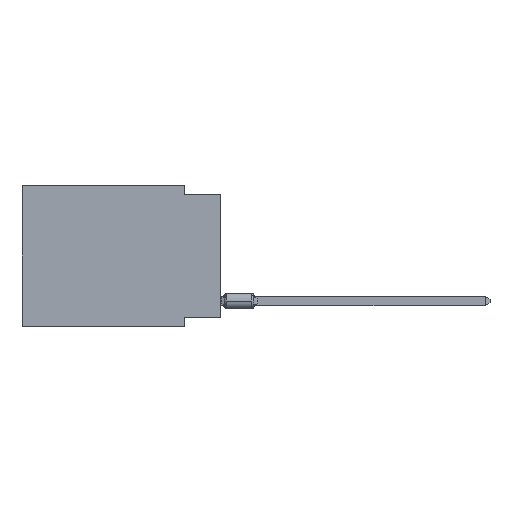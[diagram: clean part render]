
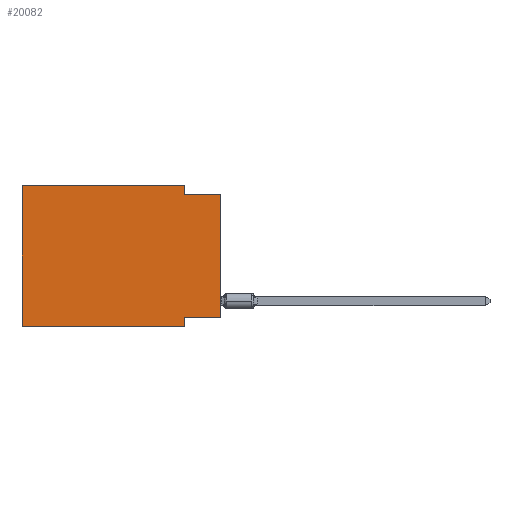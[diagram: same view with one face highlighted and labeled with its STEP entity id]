
A CAD part, left-side view. The second image highlights one B-rep face of the part: STEP entity #20082.
In plain terms, the highlighted planar face has unit normal (-1, 0, 0).
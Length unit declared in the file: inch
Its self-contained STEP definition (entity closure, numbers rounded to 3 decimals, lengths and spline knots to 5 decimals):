
#296 = VERTEX_POINT ( 'NONE', #24449 ) ;
#1430 = CARTESIAN_POINT ( 'NONE',  ( 0., 0.55, 0. ) ) ;
#1585 = ORIENTED_EDGE ( 'NONE', *, *, #33743, .F. ) ;
#2150 = CARTESIAN_POINT ( 'NONE',  ( 0., 0.1, -0.39 ) ) ;
#3085 = LINE ( 'NONE', #27768, #36129 ) ;
#3316 = ORIENTED_EDGE ( 'NONE', *, *, #31457, .F. ) ;
#4419 = CARTESIAN_POINT ( 'NONE',  ( 0., 0., -0.025 ) ) ;
#4659 = DIRECTION ( 'NONE',  ( 1., 0., 0. ) ) ;
#4661 = EDGE_CURVE ( 'NONE', #14690, #7170, #20690, .T. ) ;
#6066 = EDGE_CURVE ( 'NONE', #33749, #36734, #11482, .T. ) ;
#6223 = LINE ( 'NONE', #31396, #40293 ) ;
#7170 = VERTEX_POINT ( 'NONE', #2150 ) ;
#8730 = EDGE_LOOP ( 'NONE', ( #40315, #3316, #1585, #43874, #40571, #9997, #23531, #31334 ) ) ;
#8851 = DIRECTION ( 'NONE',  ( 0., 0., -1. ) ) ;
#9298 = LINE ( 'NONE', #12766, #36485 ) ;
#9997 = ORIENTED_EDGE ( 'NONE', *, *, #4661, .T. ) ;
#10073 = DIRECTION ( 'NONE',  ( 0., -1., 0. ) ) ;
#10293 = CARTESIAN_POINT ( 'NONE',  ( 0., 0.1, -0.365 ) ) ;
#11482 = LINE ( 'NONE', #38988, #27968 ) ;
#11809 = CARTESIAN_POINT ( 'NONE',  ( 0., 0., -0.365 ) ) ;
#12328 = VECTOR ( 'NONE', #10073, 39.37008 ) ;
#12766 = CARTESIAN_POINT ( 'NONE',  ( 0., 0.1, -0.39 ) ) ;
#13366 = CARTESIAN_POINT ( 'NONE',  ( 0., 0.1, 0. ) ) ;
#13675 = DIRECTION ( 'NONE',  ( 0., 0., -1. ) ) ;
#14138 = CARTESIAN_POINT ( 'NONE',  ( 0., 0.55, 0. ) ) ;
#14594 = FACE_OUTER_BOUND ( 'NONE', #8730, .T. ) ;
#14690 = VERTEX_POINT ( 'NONE', #22572 ) ;
#15009 = AXIS2_PLACEMENT_3D ( 'NONE', #1430, #4659, #25920 ) ;
#16118 = VERTEX_POINT ( 'NONE', #10293 ) ;
#18656 = LINE ( 'NONE', #36907, #40314 ) ;
#20082 = ADVANCED_FACE ( 'NONE', ( #14594 ), #32139, .F. ) ;
#20690 = LINE ( 'NONE', #31981, #36551 ) ;
#20991 = DIRECTION ( 'NONE',  ( 0., 0., 1. ) ) ;
#21405 = CARTESIAN_POINT ( 'NONE',  ( 0., 0., -0.025 ) ) ;
#22572 = CARTESIAN_POINT ( 'NONE',  ( 0., 0.55, -0.39 ) ) ;
#23531 = ORIENTED_EDGE ( 'NONE', *, *, #25325, .F. ) ;
#23603 = EDGE_CURVE ( 'NONE', #39385, #16118, #18656, .T. ) ;
#24449 = CARTESIAN_POINT ( 'NONE',  ( 0., 0.1, -0.025 ) ) ;
#25109 = LINE ( 'NONE', #21405, #12328 ) ;
#25325 = EDGE_CURVE ( 'NONE', #16118, #7170, #9298, .T. ) ;
#25920 = DIRECTION ( 'NONE',  ( 0., 0., -1. ) ) ;
#26837 = CARTESIAN_POINT ( 'NONE',  ( 0., 0.55, 0. ) ) ;
#27135 = VERTEX_POINT ( 'NONE', #4419 ) ;
#27327 = EDGE_CURVE ( 'NONE', #39385, #27135, #6223, .T. ) ;
#27741 = LINE ( 'NONE', #26837, #38940 ) ;
#27768 = CARTESIAN_POINT ( 'NONE',  ( 0., 0.1, 0. ) ) ;
#27968 = VECTOR ( 'NONE', #28587, 39.37008 ) ;
#28587 = DIRECTION ( 'NONE',  ( 0., -1., 0. ) ) ;
#30510 = EDGE_CURVE ( 'NONE', #14690, #33749, #27741, .T. ) ;
#31334 = ORIENTED_EDGE ( 'NONE', *, *, #23603, .F. ) ;
#31396 = CARTESIAN_POINT ( 'NONE',  ( 0., 0., 0. ) ) ;
#31457 = EDGE_CURVE ( 'NONE', #296, #27135, #25109, .T. ) ;
#31981 = CARTESIAN_POINT ( 'NONE',  ( 0., 0.55, -0.39 ) ) ;
#32139 = PLANE ( 'NONE',  #15009 ) ;
#33743 = EDGE_CURVE ( 'NONE', #36734, #296, #3085, .T. ) ;
#33749 = VERTEX_POINT ( 'NONE', #14138 ) ;
#36129 = VECTOR ( 'NONE', #13675, 39.37008 ) ;
#36485 = VECTOR ( 'NONE', #8851, 39.37008 ) ;
#36551 = VECTOR ( 'NONE', #41936, 39.37008 ) ;
#36734 = VERTEX_POINT ( 'NONE', #13366 ) ;
#36907 = CARTESIAN_POINT ( 'NONE',  ( 0., 0., -0.365 ) ) ;
#38940 = VECTOR ( 'NONE', #44849, 39.37008 ) ;
#38988 = CARTESIAN_POINT ( 'NONE',  ( 0., 0.55, 0. ) ) ;
#39385 = VERTEX_POINT ( 'NONE', #11809 ) ;
#40293 = VECTOR ( 'NONE', #20991, 39.37008 ) ;
#40314 = VECTOR ( 'NONE', #43140, 39.37008 ) ;
#40315 = ORIENTED_EDGE ( 'NONE', *, *, #27327, .T. ) ;
#40571 = ORIENTED_EDGE ( 'NONE', *, *, #30510, .F. ) ;
#41936 = DIRECTION ( 'NONE',  ( 0., -1., 0. ) ) ;
#43140 = DIRECTION ( 'NONE',  ( 0., 1., 0. ) ) ;
#43874 = ORIENTED_EDGE ( 'NONE', *, *, #6066, .F. ) ;
#44849 = DIRECTION ( 'NONE',  ( 0., 0., 1. ) ) ;
